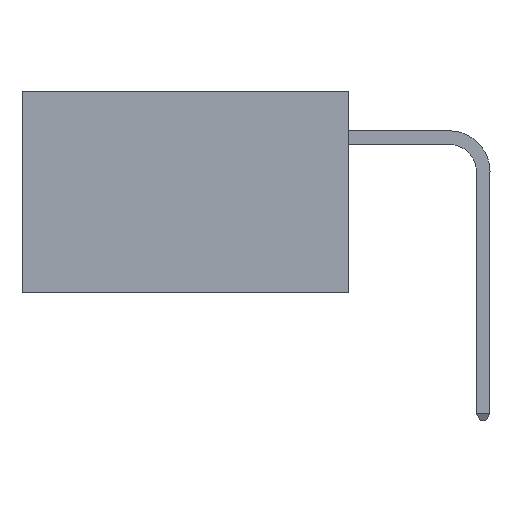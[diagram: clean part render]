
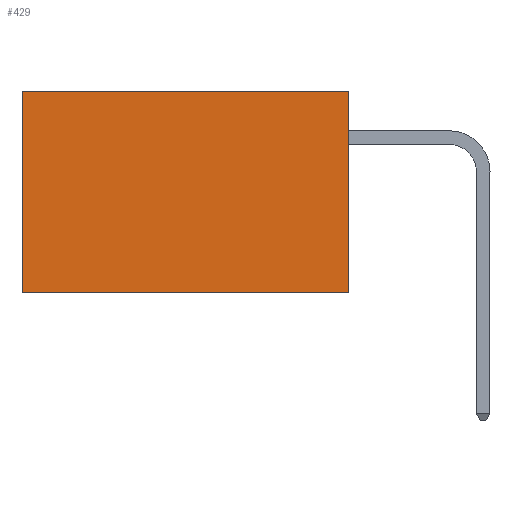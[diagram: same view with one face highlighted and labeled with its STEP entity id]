
A CAD part, left-side view. The second image highlights one B-rep face of the part: STEP entity #429.
In plain terms, the highlighted planar face has unit normal (-1, 0, 0).
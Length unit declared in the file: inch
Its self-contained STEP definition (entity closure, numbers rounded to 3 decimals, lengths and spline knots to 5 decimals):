
#429 = ADVANCED_FACE ( 'NONE', ( #11626 ), #6029, .F. ) ;
#1729 = EDGE_CURVE ( 'NONE', #5820, #7563, #10352, .T. ) ;
#1939 = ORIENTED_EDGE ( 'NONE', *, *, #11423, .F. ) ;
#2103 = CARTESIAN_POINT ( 'NONE',  ( 0.2875, 0., -0.37 ) ) ;
#2835 = DIRECTION ( 'NONE',  ( 0., 1., 0. ) ) ;
#3113 = CARTESIAN_POINT ( 'NONE',  ( 0.2875, 0.6, 0. ) ) ;
#4375 = CARTESIAN_POINT ( 'NONE',  ( 0.2875, 0., 0. ) ) ;
#4638 = VERTEX_POINT ( 'NONE', #3113 ) ;
#4679 = ORIENTED_EDGE ( 'NONE', *, *, #12854, .T. ) ;
#4825 = DIRECTION ( 'NONE',  ( 0., 0., -1. ) ) ;
#5820 = VERTEX_POINT ( 'NONE', #11999 ) ;
#5871 = CARTESIAN_POINT ( 'NONE',  ( 0.2875, 0.6, -0.37 ) ) ;
#6029 = PLANE ( 'NONE',  #8062 ) ;
#6121 = DIRECTION ( 'NONE',  ( 1., 0., 0. ) ) ;
#6953 = DIRECTION ( 'NONE',  ( 0., 0., -1. ) ) ;
#7524 = DIRECTION ( 'NONE',  ( 0., 0., -1. ) ) ;
#7559 = ORIENTED_EDGE ( 'NONE', *, *, #10198, .T. ) ;
#7563 = VERTEX_POINT ( 'NONE', #5871 ) ;
#8062 = AXIS2_PLACEMENT_3D ( 'NONE', #9142, #6121, #6953 ) ;
#8254 = VECTOR ( 'NONE', #4825, 39.37008 ) ;
#8264 = ORIENTED_EDGE ( 'NONE', *, *, #1729, .F. ) ;
#8579 = VERTEX_POINT ( 'NONE', #10531 ) ;
#9130 = LINE ( 'NONE', #4375, #11765 ) ;
#9142 = CARTESIAN_POINT ( 'NONE',  ( 0.2875, 0., 0. ) ) ;
#9471 = EDGE_LOOP ( 'NONE', ( #4679, #8264, #1939, #7559 ) ) ;
#9581 = VECTOR ( 'NONE', #2835, 39.37008 ) ;
#9801 = VECTOR ( 'NONE', #12042, 39.37008 ) ;
#10198 = EDGE_CURVE ( 'NONE', #8579, #4638, #11652, .T. ) ;
#10352 = LINE ( 'NONE', #2103, #9801 ) ;
#10531 = CARTESIAN_POINT ( 'NONE',  ( 0.2875, 0., 0. ) ) ;
#10587 = CARTESIAN_POINT ( 'NONE',  ( 0.2875, 0.6, 0. ) ) ;
#11423 = EDGE_CURVE ( 'NONE', #8579, #5820, #9130, .T. ) ;
#11626 = FACE_OUTER_BOUND ( 'NONE', #9471, .T. ) ;
#11646 = CARTESIAN_POINT ( 'NONE',  ( 0.2875, 0., 0. ) ) ;
#11652 = LINE ( 'NONE', #11646, #9581 ) ;
#11765 = VECTOR ( 'NONE', #7524, 39.37008 ) ;
#11999 = CARTESIAN_POINT ( 'NONE',  ( 0.2875, 0., -0.37 ) ) ;
#12042 = DIRECTION ( 'NONE',  ( 0., 1., 0. ) ) ;
#12854 = EDGE_CURVE ( 'NONE', #4638, #7563, #12893, .T. ) ;
#12893 = LINE ( 'NONE', #10587, #8254 ) ;
